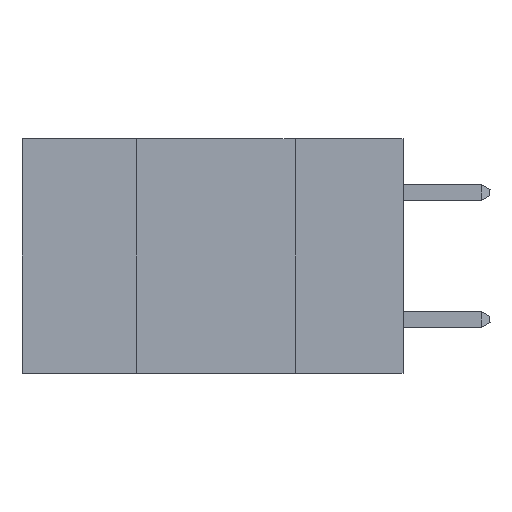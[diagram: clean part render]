
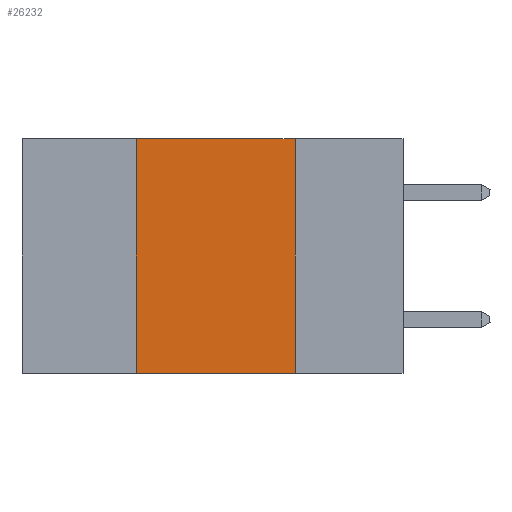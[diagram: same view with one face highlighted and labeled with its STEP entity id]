
A CAD part, left-side view. The second image highlights one B-rep face of the part: STEP entity #26232.
In plain terms, the highlighted planar face has unit normal (-1, 0, 0).
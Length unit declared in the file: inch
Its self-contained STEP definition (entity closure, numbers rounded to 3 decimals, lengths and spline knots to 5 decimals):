
#155 = LINE ( 'NONE', #25392, #31306 ) ;
#1461 = EDGE_CURVE ( 'NONE', #26711, #26571, #155, .T. ) ;
#1815 = FACE_OUTER_BOUND ( 'NONE', #28665, .T. ) ;
#2448 = VECTOR ( 'NONE', #14858, 39.37008 ) ;
#9998 = CARTESIAN_POINT ( 'NONE',  ( 0., 0.42, 0. ) ) ;
#10110 = VECTOR ( 'NONE', #26425, 39.37008 ) ;
#10403 = CARTESIAN_POINT ( 'NONE',  ( 0., 0.42, 0. ) ) ;
#10769 = ORIENTED_EDGE ( 'NONE', *, *, #1461, .F. ) ;
#13039 = EDGE_CURVE ( 'NONE', #17655, #26711, #20142, .T. ) ;
#13518 = EDGE_CURVE ( 'NONE', #17655, #19714, #13570, .T. ) ;
#13570 = LINE ( 'NONE', #14254, #10110 ) ;
#14097 = EDGE_CURVE ( 'NONE', #26571, #19714, #30107, .T. ) ;
#14254 = CARTESIAN_POINT ( 'NONE',  ( 0., 0.6, -0.37 ) ) ;
#14761 = AXIS2_PLACEMENT_3D ( 'NONE', #15377, #17851, #15157 ) ;
#14836 = ORIENTED_EDGE ( 'NONE', *, *, #13039, .F. ) ;
#14858 = DIRECTION ( 'NONE',  ( 0., 0., 1. ) ) ;
#15109 = ORIENTED_EDGE ( 'NONE', *, *, #14097, .F. ) ;
#15157 = DIRECTION ( 'NONE',  ( 0., 0., -1. ) ) ;
#15377 = CARTESIAN_POINT ( 'NONE',  ( 0., 0.6, 0. ) ) ;
#17647 = PLANE ( 'NONE',  #14761 ) ;
#17655 = VERTEX_POINT ( 'NONE', #18605 ) ;
#17851 = DIRECTION ( 'NONE',  ( 1., 0., 0. ) ) ;
#18605 = CARTESIAN_POINT ( 'NONE',  ( 0., 0.42, -0.37 ) ) ;
#18655 = DIRECTION ( 'NONE',  ( 0., 0., -1. ) ) ;
#19714 = VERTEX_POINT ( 'NONE', #26851 ) ;
#20142 = LINE ( 'NONE', #9998, #2448 ) ;
#20203 = DIRECTION ( 'NONE',  ( 0., -1., 0. ) ) ;
#22378 = ORIENTED_EDGE ( 'NONE', *, *, #13518, .T. ) ;
#23688 = CARTESIAN_POINT ( 'NONE',  ( 0., 0.17, 0. ) ) ;
#25392 = CARTESIAN_POINT ( 'NONE',  ( 0., 0.6, 0. ) ) ;
#25482 = VECTOR ( 'NONE', #18655, 39.37008 ) ;
#26232 = ADVANCED_FACE ( 'NONE', ( #1815 ), #17647, .F. ) ;
#26425 = DIRECTION ( 'NONE',  ( 0., -1., 0. ) ) ;
#26571 = VERTEX_POINT ( 'NONE', #29606 ) ;
#26711 = VERTEX_POINT ( 'NONE', #10403 ) ;
#26851 = CARTESIAN_POINT ( 'NONE',  ( 0., 0.17, -0.37 ) ) ;
#28665 = EDGE_LOOP ( 'NONE', ( #15109, #10769, #14836, #22378 ) ) ;
#29606 = CARTESIAN_POINT ( 'NONE',  ( 0., 0.17, 0. ) ) ;
#30107 = LINE ( 'NONE', #23688, #25482 ) ;
#31306 = VECTOR ( 'NONE', #20203, 39.37008 ) ;
